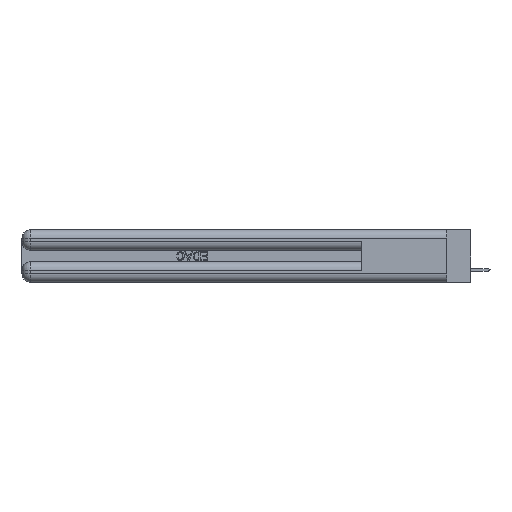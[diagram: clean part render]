
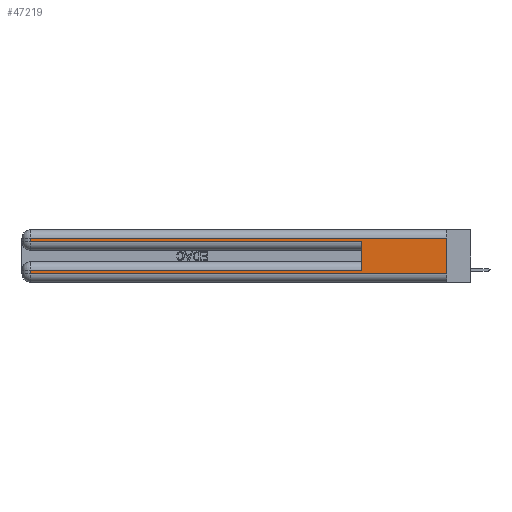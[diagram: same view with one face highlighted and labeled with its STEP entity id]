
A CAD part, left-side view. The second image highlights one B-rep face of the part: STEP entity #47219.
In plain terms, the highlighted planar face has unit normal (-1, 0, 0).
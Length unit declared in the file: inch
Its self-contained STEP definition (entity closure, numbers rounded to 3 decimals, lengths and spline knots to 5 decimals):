
#1391 = EDGE_CURVE ( 'NONE', #49929, #46358, #5806, .T. ) ;
#1773 = VERTEX_POINT ( 'NONE', #48222 ) ;
#1975 = DIRECTION ( 'NONE',  ( 0., 0., -1. ) ) ;
#2058 = ORIENTED_EDGE ( 'NONE', *, *, #1391, .F. ) ;
#2527 = VECTOR ( 'NONE', #34434, 39.37008 ) ;
#2850 = DIRECTION ( 'NONE',  ( 0., 0., 1. ) ) ;
#4352 = VERTEX_POINT ( 'NONE', #22301 ) ;
#5103 = PLANE ( 'NONE',  #42593 ) ;
#5635 = LINE ( 'NONE', #24299, #21555 ) ;
#5806 = LINE ( 'NONE', #48551, #42282 ) ;
#5814 = VECTOR ( 'NONE', #46343, 39.37008 ) ;
#8658 = EDGE_CURVE ( 'NONE', #39041, #9977, #5635, .T. ) ;
#9958 = EDGE_CURVE ( 'NONE', #31817, #4352, #9998, .T. ) ;
#9977 = VERTEX_POINT ( 'NONE', #10728 ) ;
#9998 = LINE ( 'NONE', #34517, #16703 ) ;
#10092 = CARTESIAN_POINT ( 'NONE',  ( 0., 2.94, 0.285 ) ) ;
#10728 = CARTESIAN_POINT ( 'NONE',  ( 0., 2.94, 0.085 ) ) ;
#10779 = LINE ( 'NONE', #25899, #41719 ) ;
#13282 = DIRECTION ( 'NONE',  ( 1., 0., 0. ) ) ;
#16703 = VECTOR ( 'NONE', #45304, 39.37008 ) ;
#20859 = VECTOR ( 'NONE', #37834, 39.37008 ) ;
#21555 = VECTOR ( 'NONE', #24554, 39.37008 ) ;
#22301 = CARTESIAN_POINT ( 'NONE',  ( 0., 0.6, 0.285 ) ) ;
#23259 = CARTESIAN_POINT ( 'NONE',  ( 0., 0., 0.31 ) ) ;
#24299 = CARTESIAN_POINT ( 'NONE',  ( 0., 0., 0.085 ) ) ;
#24554 = DIRECTION ( 'NONE',  ( 0., 1., 0. ) ) ;
#25267 = VERTEX_POINT ( 'NONE', #47441 ) ;
#25543 = LINE ( 'NONE', #48855, #20859 ) ;
#25899 = CARTESIAN_POINT ( 'NONE',  ( 0., 0.6, 0.145 ) ) ;
#26233 = EDGE_CURVE ( 'NONE', #1773, #31817, #30330, .T. ) ;
#26404 = ORIENTED_EDGE ( 'NONE', *, *, #26233, .T. ) ;
#26736 = ORIENTED_EDGE ( 'NONE', *, *, #48231, .F. ) ;
#27968 = ORIENTED_EDGE ( 'NONE', *, *, #8658, .T. ) ;
#28146 = CARTESIAN_POINT ( 'NONE',  ( 0., 0., 0.37 ) ) ;
#29887 = EDGE_CURVE ( 'NONE', #9977, #25267, #25543, .T. ) ;
#30104 = CARTESIAN_POINT ( 'NONE',  ( 0., 0., 0.06 ) ) ;
#30302 = ORIENTED_EDGE ( 'NONE', *, *, #9958, .T. ) ;
#30330 = LINE ( 'NONE', #44954, #33821 ) ;
#30341 = LINE ( 'NONE', #30104, #2527 ) ;
#31525 = EDGE_CURVE ( 'NONE', #25267, #46358, #30341, .T. ) ;
#31817 = VERTEX_POINT ( 'NONE', #10092 ) ;
#32016 = CARTESIAN_POINT ( 'NONE',  ( 0., 0.6, 0.085 ) ) ;
#33821 = VECTOR ( 'NONE', #45974, 39.37008 ) ;
#34434 = DIRECTION ( 'NONE',  ( 0., -1., 0. ) ) ;
#34517 = CARTESIAN_POINT ( 'NONE',  ( 0., 0., 0.285 ) ) ;
#35033 = CARTESIAN_POINT ( 'NONE',  ( 0., 0., 0.31 ) ) ;
#37156 = ORIENTED_EDGE ( 'NONE', *, *, #29887, .T. ) ;
#37834 = DIRECTION ( 'NONE',  ( 0., 0., -1. ) ) ;
#38655 = LINE ( 'NONE', #23259, #5814 ) ;
#39041 = VERTEX_POINT ( 'NONE', #32016 ) ;
#40497 = ORIENTED_EDGE ( 'NONE', *, *, #47070, .T. ) ;
#41107 = ORIENTED_EDGE ( 'NONE', *, *, #31525, .T. ) ;
#41719 = VECTOR ( 'NONE', #2850, 39.37008 ) ;
#42238 = EDGE_LOOP ( 'NONE', ( #2058, #40497, #26404, #30302, #26736, #27968, #37156, #41107 ) ) ;
#42282 = VECTOR ( 'NONE', #1975, 39.37008 ) ;
#42593 = AXIS2_PLACEMENT_3D ( 'NONE', #28146, #13282, #43490 ) ;
#43490 = DIRECTION ( 'NONE',  ( 0., 0., -1. ) ) ;
#43883 = CARTESIAN_POINT ( 'NONE',  ( 0., 0., 0.06 ) ) ;
#44534 = FACE_OUTER_BOUND ( 'NONE', #42238, .T. ) ;
#44954 = CARTESIAN_POINT ( 'NONE',  ( 0., 2.94, 0.37 ) ) ;
#45304 = DIRECTION ( 'NONE',  ( 0., -1., 0. ) ) ;
#45974 = DIRECTION ( 'NONE',  ( 0., 0., -1. ) ) ;
#46343 = DIRECTION ( 'NONE',  ( 0., 1., 0. ) ) ;
#46358 = VERTEX_POINT ( 'NONE', #43883 ) ;
#47070 = EDGE_CURVE ( 'NONE', #49929, #1773, #38655, .T. ) ;
#47219 = ADVANCED_FACE ( 'NONE', ( #44534 ), #5103, .F. ) ;
#47441 = CARTESIAN_POINT ( 'NONE',  ( 0., 2.94, 0.06 ) ) ;
#48222 = CARTESIAN_POINT ( 'NONE',  ( 0., 2.94, 0.31 ) ) ;
#48231 = EDGE_CURVE ( 'NONE', #39041, #4352, #10779, .T. ) ;
#48551 = CARTESIAN_POINT ( 'NONE',  ( 0., 0., 0.37 ) ) ;
#48855 = CARTESIAN_POINT ( 'NONE',  ( 0., 2.94, 0.37 ) ) ;
#49929 = VERTEX_POINT ( 'NONE', #35033 ) ;
